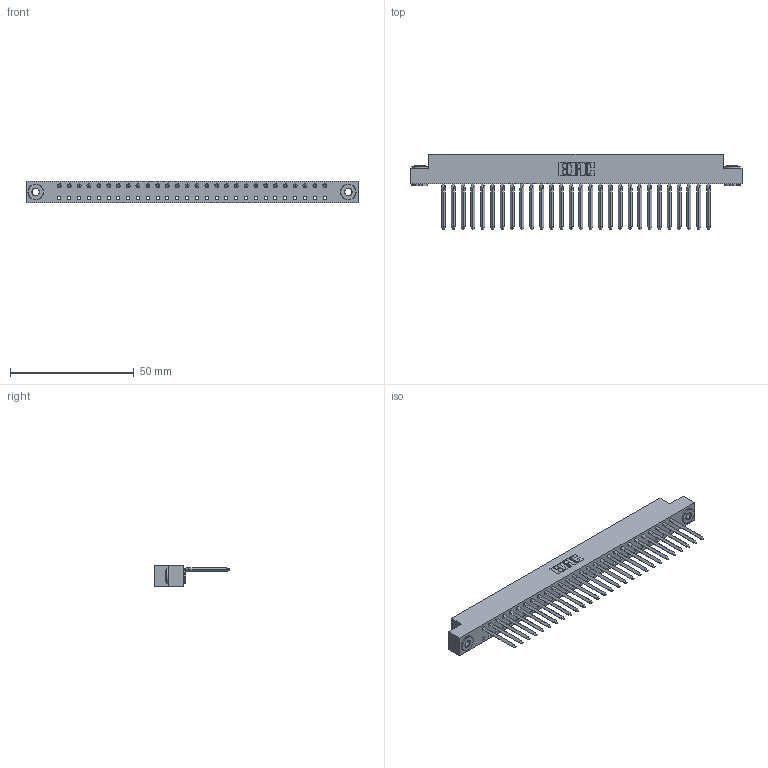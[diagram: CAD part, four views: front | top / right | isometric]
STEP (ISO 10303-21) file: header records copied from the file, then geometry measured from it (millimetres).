
FILE_DESCRIPTION (( 'STEP AP203' ), '1' );
FILE_NAME ('338-028-541-103.STEP', '2020-03-24T17:58:59', ( '' ), ( '' ), 'SwSTEP 2.0', 'SolidWorks 2016', '' );
FILE_SCHEMA (( 'CONFIG_CONTROL_DESIGN' ));
Length unit declared in the file: inch
Products named in the file (4): 338-210-001_338-210-028-004; 345-250-002_345-250-002-102; 338-290-001_541; 338-028-541-103
Assembly tree (31 placements, depth 2):
  338-028-541-103
    338-210-001_338-210-028-004
    338-290-001_541  x28
    345-250-002_345-250-002-102  x2
Bounding box: 133.96 x 30.56 x 8.71 mm (x, y, z)
Volume: 9401.7 mm3; surface area: 15650 mm2
Topology: 31 solids, 31 shells, 2750 faces, 7559 edges, 4830 vertices
Faces by surface type: plane 1894, cylinder 736, bspline 112, cone 8
Entity records: 56177 total; most frequent: CARTESIAN_POINT 11233, ORIENTED_EDGE 9480, DIRECTION 8869, EDGE_CURVE 4740, VECTOR 3537, LINE 3537, VERTEX_POINT 3078, AXIS2_PLACEMENT_3D 2666
